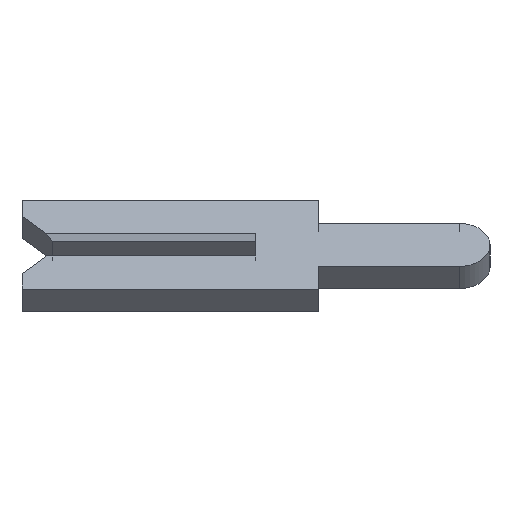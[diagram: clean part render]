
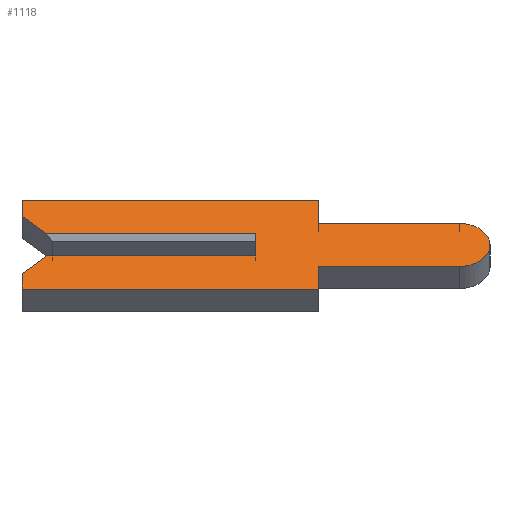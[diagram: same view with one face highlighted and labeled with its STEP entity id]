
A CAD part, left-side view. The second image highlights one B-rep face of the part: STEP entity #1118.
In plain terms, the highlighted face is planar.
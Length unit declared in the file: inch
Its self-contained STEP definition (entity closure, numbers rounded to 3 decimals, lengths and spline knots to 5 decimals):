
#20 = EDGE_LOOP ( 'NONE', ( #132, #863, #725, #755, #478, #297, #279, #697, #223, #485, #154, #1188, #347, #772 ) ) ;
#23 = AXIS2_PLACEMENT_3D ( 'NONE', #1129, #459, #728 ) ;
#35 = LINE ( 'NONE', #206, #606 ) ;
#46 = AXIS2_PLACEMENT_3D ( 'NONE', #388, #1154, #675 ) ;
#48 = VECTOR ( 'NONE', #403, 39.37008 ) ;
#63 = DIRECTION ( 'NONE',  ( 0., -1., 0. ) ) ;
#65 = LINE ( 'NONE', #383, #690 ) ;
#76 = DIRECTION ( 'NONE',  ( 0., -1., 0. ) ) ;
#97 = CARTESIAN_POINT ( 'NONE',  ( -0.01, -0.1305, -0.0195 ) ) ;
#102 = VERTEX_POINT ( 'NONE', #612 ) ;
#127 = VERTEX_POINT ( 'NONE', #137 ) ;
#132 = ORIENTED_EDGE ( 'NONE', *, *, #531, .T. ) ;
#136 = LINE ( 'NONE', #283, #48 ) ;
#137 = CARTESIAN_POINT ( 'NONE',  ( -0.01, -0.04, -0.0195 ) ) ;
#146 = EDGE_CURVE ( 'NONE', #252, #738, #760, .T. ) ;
#154 = ORIENTED_EDGE ( 'NONE', *, *, #648, .F. ) ;
#186 = DIRECTION ( 'NONE',  ( 0., 0.707, 0.707 ) ) ;
#206 = CARTESIAN_POINT ( 'NONE',  ( -0.01, 0.1305, 0.0065 ) ) ;
#212 = LINE ( 'NONE', #475, #811 ) ;
#223 = ORIENTED_EDGE ( 'NONE', *, *, #716, .F. ) ;
#241 = LINE ( 'NONE', #369, #686 ) ;
#243 = VERTEX_POINT ( 'NONE', #524 ) ;
#252 = VERTEX_POINT ( 'NONE', #337 ) ;
#270 = LINE ( 'NONE', #1199, #1130 ) ;
#271 = EDGE_CURVE ( 'NONE', #1189, #583, #270, .T. ) ;
#279 = ORIENTED_EDGE ( 'NONE', *, *, #406, .F. ) ;
#283 = CARTESIAN_POINT ( 'NONE',  ( -0.01, 0.15, -0.04 ) ) ;
#297 = ORIENTED_EDGE ( 'NONE', *, *, #489, .F. ) ;
#306 = VECTOR ( 'NONE', #76, 39.37008 ) ;
#316 = VERTEX_POINT ( 'NONE', #747 ) ;
#325 = VECTOR ( 'NONE', #395, 39.37008 ) ;
#327 = VERTEX_POINT ( 'NONE', #1053 ) ;
#328 = DIRECTION ( 'NONE',  ( 0., -1., 0. ) ) ;
#337 = CARTESIAN_POINT ( 'NONE',  ( -0.01, 0.15, -0.04 ) ) ;
#347 = ORIENTED_EDGE ( 'NONE', *, *, #740, .F. ) ;
#358 = EDGE_CURVE ( 'NONE', #327, #316, #843, .T. ) ;
#360 = CARTESIAN_POINT ( 'NONE',  ( -0.01, -0.04, -0.04 ) ) ;
#369 = CARTESIAN_POINT ( 'NONE',  ( -0.01, -0.04, -0.04 ) ) ;
#375 = CARTESIAN_POINT ( 'NONE',  ( -0.01, 0., 0.01 ) ) ;
#383 = CARTESIAN_POINT ( 'NONE',  ( -0.01, -0.04, 0.04 ) ) ;
#388 = CARTESIAN_POINT ( 'NONE',  ( -0.01, -0.1305, 0. ) ) ;
#395 = DIRECTION ( 'NONE',  ( 0., -1., 0. ) ) ;
#398 = DIRECTION ( 'NONE',  ( 0., 0., -1. ) ) ;
#403 = DIRECTION ( 'NONE',  ( 0., 1., 0. ) ) ;
#406 = EDGE_CURVE ( 'NONE', #127, #999, #241, .T. ) ;
#410 = EDGE_CURVE ( 'NONE', #474, #127, #212, .T. ) ;
#426 = CARTESIAN_POINT ( 'NONE',  ( -0.01, 0.15, -0.026 ) ) ;
#444 = LINE ( 'NONE', #1246, #860 ) ;
#459 = DIRECTION ( 'NONE',  ( 1., 0., 0. ) ) ;
#473 = LINE ( 'NONE', #1224, #560 ) ;
#474 = VERTEX_POINT ( 'NONE', #97 ) ;
#475 = CARTESIAN_POINT ( 'NONE',  ( -0.01, -0.04, -0.0195 ) ) ;
#478 = ORIENTED_EDGE ( 'NONE', *, *, #146, .F. ) ;
#481 = CARTESIAN_POINT ( 'NONE',  ( -0.01, 0.1305, -0.0065 ) ) ;
#485 = ORIENTED_EDGE ( 'NONE', *, *, #358, .F. ) ;
#489 = EDGE_CURVE ( 'NONE', #999, #252, #136, .T. ) ;
#493 = DIRECTION ( 'NONE',  ( 0., 0., 1. ) ) ;
#511 = VECTOR ( 'NONE', #1107, 39.37008 ) ;
#524 = CARTESIAN_POINT ( 'NONE',  ( -0.01, 0.15, 0.04 ) ) ;
#531 = EDGE_CURVE ( 'NONE', #102, #1124, #991, .T. ) ;
#560 = VECTOR ( 'NONE', #63, 39.37008 ) ;
#563 = PLANE ( 'NONE',  #23 ) ;
#575 = CARTESIAN_POINT ( 'NONE',  ( -0.01, 0., 0.0065 ) ) ;
#579 = VECTOR ( 'NONE', #776, 39.37008 ) ;
#580 = CARTESIAN_POINT ( 'NONE',  ( -0.01, 0.15, -0.026 ) ) ;
#583 = VERTEX_POINT ( 'NONE', #1169 ) ;
#597 = EDGE_CURVE ( 'NONE', #738, #1189, #768, .T. ) ;
#606 = VECTOR ( 'NONE', #186, 39.37008 ) ;
#612 = CARTESIAN_POINT ( 'NONE',  ( -0.01, 0.134, 0.01 ) ) ;
#632 = CARTESIAN_POINT ( 'NONE',  ( -0.01, 0.134, -0.01 ) ) ;
#648 = EDGE_CURVE ( 'NONE', #1219, #327, #65, .T. ) ;
#653 = EDGE_CURVE ( 'NONE', #583, #1124, #887, .T. ) ;
#671 = CARTESIAN_POINT ( 'NONE',  ( -0.01, 0.15, 0.026 ) ) ;
#675 = DIRECTION ( 'NONE',  ( 0., 0., -1. ) ) ;
#686 = VECTOR ( 'NONE', #398, 39.37008 ) ;
#690 = VECTOR ( 'NONE', #773, 39.37008 ) ;
#697 = ORIENTED_EDGE ( 'NONE', *, *, #410, .F. ) ;
#716 = EDGE_CURVE ( 'NONE', #316, #474, #1121, .T. ) ;
#719 = VERTEX_POINT ( 'NONE', #671 ) ;
#725 = ORIENTED_EDGE ( 'NONE', *, *, #271, .F. ) ;
#728 = DIRECTION ( 'NONE',  ( 0., 0., -1. ) ) ;
#738 = VERTEX_POINT ( 'NONE', #580 ) ;
#740 = EDGE_CURVE ( 'NONE', #719, #243, #444, .T. ) ;
#747 = CARTESIAN_POINT ( 'NONE',  ( -0.01, -0.1305, 0.0195 ) ) ;
#751 = CARTESIAN_POINT ( 'NONE',  ( -0.01, -0.04, 0.0195 ) ) ;
#755 = ORIENTED_EDGE ( 'NONE', *, *, #597, .F. ) ;
#760 = LINE ( 'NONE', #426, #511 ) ;
#768 = LINE ( 'NONE', #481, #579 ) ;
#772 = ORIENTED_EDGE ( 'NONE', *, *, #785, .F. ) ;
#773 = DIRECTION ( 'NONE',  ( 0., 0., -1. ) ) ;
#776 = DIRECTION ( 'NONE',  ( 0., -0.707, 0.707 ) ) ;
#785 = EDGE_CURVE ( 'NONE', #102, #719, #35, .T. ) ;
#811 = VECTOR ( 'NONE', #1067, 39.37008 ) ;
#843 = LINE ( 'NONE', #751, #306 ) ;
#860 = VECTOR ( 'NONE', #493, 39.37008 ) ;
#863 = ORIENTED_EDGE ( 'NONE', *, *, #653, .F. ) ;
#870 = DIRECTION ( 'NONE',  ( 0., 0., 1. ) ) ;
#887 = LINE ( 'NONE', #575, #1061 ) ;
#934 = CARTESIAN_POINT ( 'NONE',  ( -0.01, -0.04, 0.04 ) ) ;
#950 = CARTESIAN_POINT ( 'NONE',  ( -0.01, 0.15, 0.01 ) ) ;
#991 = LINE ( 'NONE', #950, #325 ) ;
#999 = VERTEX_POINT ( 'NONE', #360 ) ;
#1046 = EDGE_CURVE ( 'NONE', #243, #1219, #473, .T. ) ;
#1053 = CARTESIAN_POINT ( 'NONE',  ( -0.01, -0.04, 0.0195 ) ) ;
#1061 = VECTOR ( 'NONE', #870, 39.37008 ) ;
#1067 = DIRECTION ( 'NONE',  ( 0., 1., 0. ) ) ;
#1107 = DIRECTION ( 'NONE',  ( 0., 0., 1. ) ) ;
#1118 = ADVANCED_FACE ( 'NONE', ( #1131 ), #563, .F. ) ;
#1121 = CIRCLE ( 'NONE', #46, 0.0195 ) ;
#1124 = VERTEX_POINT ( 'NONE', #375 ) ;
#1129 = CARTESIAN_POINT ( 'NONE',  ( -0.01, -0.1305, 0. ) ) ;
#1130 = VECTOR ( 'NONE', #328, 39.37008 ) ;
#1131 = FACE_OUTER_BOUND ( 'NONE', #20, .T. ) ;
#1154 = DIRECTION ( 'NONE',  ( 1., 0., 0. ) ) ;
#1169 = CARTESIAN_POINT ( 'NONE',  ( -0.01, 0., -0.01 ) ) ;
#1188 = ORIENTED_EDGE ( 'NONE', *, *, #1046, .F. ) ;
#1189 = VERTEX_POINT ( 'NONE', #632 ) ;
#1199 = CARTESIAN_POINT ( 'NONE',  ( -0.01, -0.1305, -0.01 ) ) ;
#1219 = VERTEX_POINT ( 'NONE', #934 ) ;
#1224 = CARTESIAN_POINT ( 'NONE',  ( -0.01, 0.15, 0.04 ) ) ;
#1246 = CARTESIAN_POINT ( 'NONE',  ( -0.01, 0.15, 0.026 ) ) ;
